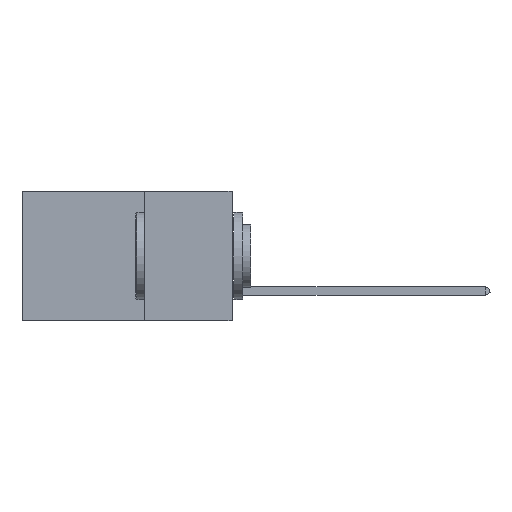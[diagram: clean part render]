
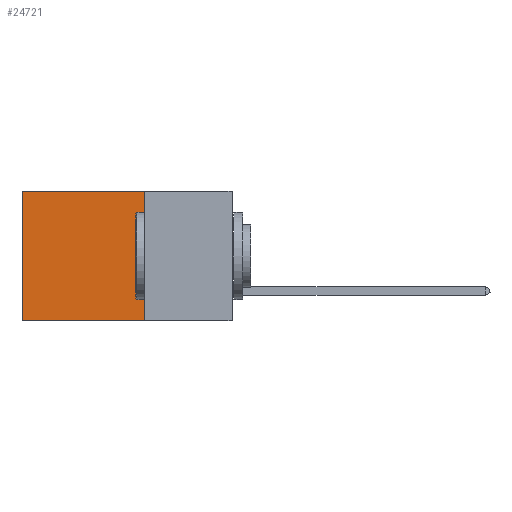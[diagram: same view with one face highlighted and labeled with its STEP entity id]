
A CAD part, left-side view. The second image highlights one B-rep face of the part: STEP entity #24721.
In plain terms, the highlighted planar face has unit normal (-1, 0, 0).
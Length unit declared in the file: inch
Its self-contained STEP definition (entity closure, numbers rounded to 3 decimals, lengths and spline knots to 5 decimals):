
#191 = CARTESIAN_POINT ( 'NONE',  ( 0.2875, 0.25, 0. ) ) ;
#423 = DIRECTION ( 'NONE',  ( 1., 0., 0. ) ) ;
#866 = CARTESIAN_POINT ( 'NONE',  ( 0.2875, 0.6, -0.37 ) ) ;
#2225 = VERTEX_POINT ( 'NONE', #866 ) ;
#4797 = VECTOR ( 'NONE', #7162, 39.37008 ) ;
#5172 = EDGE_CURVE ( 'NONE', #27445, #2225, #9384, .T. ) ;
#7162 = DIRECTION ( 'NONE',  ( 0., 1., 0. ) ) ;
#7227 = CARTESIAN_POINT ( 'NONE',  ( 0.2875, 0.25, -0.37 ) ) ;
#8149 = DIRECTION ( 'NONE',  ( 0., 0., -1. ) ) ;
#8183 = LINE ( 'NONE', #22756, #4797 ) ;
#8260 = ORIENTED_EDGE ( 'NONE', *, *, #5172, .T. ) ;
#9173 = VERTEX_POINT ( 'NONE', #16524 ) ;
#9384 = LINE ( 'NONE', #20377, #11063 ) ;
#11063 = VECTOR ( 'NONE', #22734, 39.37008 ) ;
#15044 = VECTOR ( 'NONE', #35179, 39.37008 ) ;
#15092 = EDGE_CURVE ( 'NONE', #9173, #27445, #8183, .T. ) ;
#16183 = EDGE_CURVE ( 'NONE', #22960, #2225, #27294, .T. ) ;
#16524 = CARTESIAN_POINT ( 'NONE',  ( 0.2875, 0.25, 0. ) ) ;
#18499 = FACE_OUTER_BOUND ( 'NONE', #25286, .T. ) ;
#20072 = ORIENTED_EDGE ( 'NONE', *, *, #16183, .F. ) ;
#20377 = CARTESIAN_POINT ( 'NONE',  ( 0.2875, 0.6, 0. ) ) ;
#22734 = DIRECTION ( 'NONE',  ( 0., 0., -1. ) ) ;
#22756 = CARTESIAN_POINT ( 'NONE',  ( 0.2875, 0.25, 0. ) ) ;
#22960 = VERTEX_POINT ( 'NONE', #7227 ) ;
#23373 = DIRECTION ( 'NONE',  ( 0., 1., 0. ) ) ;
#24721 = ADVANCED_FACE ( 'NONE', ( #18499 ), #32918, .F. ) ;
#25214 = ORIENTED_EDGE ( 'NONE', *, *, #15092, .T. ) ;
#25286 = EDGE_LOOP ( 'NONE', ( #8260, #20072, #29832, #25214 ) ) ;
#26381 = CARTESIAN_POINT ( 'NONE',  ( 0.2875, 0.25, -0.37 ) ) ;
#27288 = CARTESIAN_POINT ( 'NONE',  ( 0.2875, 0.6, 0. ) ) ;
#27294 = LINE ( 'NONE', #26381, #32077 ) ;
#27445 = VERTEX_POINT ( 'NONE', #27288 ) ;
#29438 = CARTESIAN_POINT ( 'NONE',  ( 0.2875, 0.25, 0. ) ) ;
#29586 = LINE ( 'NONE', #29438, #15044 ) ;
#29730 = EDGE_CURVE ( 'NONE', #9173, #22960, #29586, .T. ) ;
#29832 = ORIENTED_EDGE ( 'NONE', *, *, #29730, .F. ) ;
#32077 = VECTOR ( 'NONE', #23373, 39.37008 ) ;
#32404 = AXIS2_PLACEMENT_3D ( 'NONE', #191, #423, #8149 ) ;
#32918 = PLANE ( 'NONE',  #32404 ) ;
#35179 = DIRECTION ( 'NONE',  ( 0., 0., -1. ) ) ;
